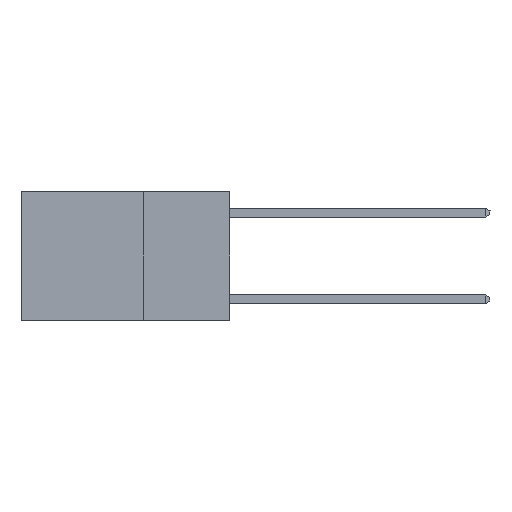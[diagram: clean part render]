
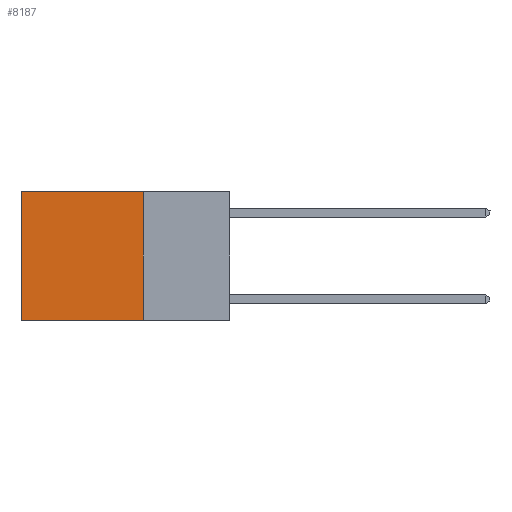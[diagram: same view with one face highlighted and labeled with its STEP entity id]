
A CAD part, left-side view. The second image highlights one B-rep face of the part: STEP entity #8187.
In plain terms, the highlighted planar face has unit normal (-1, 0, 0).
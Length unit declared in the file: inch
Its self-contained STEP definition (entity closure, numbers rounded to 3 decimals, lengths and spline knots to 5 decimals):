
#231 = EDGE_CURVE ( 'NONE', #16517, #11015, #27990, .T. ) ;
#1372 = CARTESIAN_POINT ( 'NONE',  ( 0.2625, 0.6, 0. ) ) ;
#1393 = FACE_OUTER_BOUND ( 'NONE', #3241, .T. ) ;
#1765 = DIRECTION ( 'NONE',  ( 0., 0., -1. ) ) ;
#2202 = CARTESIAN_POINT ( 'NONE',  ( 0.2625, 0.25, 0. ) ) ;
#3241 = EDGE_LOOP ( 'NONE', ( #26690, #14822, #8175, #23675 ) ) ;
#3537 = DIRECTION ( 'NONE',  ( 1., 0., 0. ) ) ;
#3926 = LINE ( 'NONE', #11166, #18707 ) ;
#4234 = DIRECTION ( 'NONE',  ( 0., 1., 0. ) ) ;
#4394 = LINE ( 'NONE', #10884, #12597 ) ;
#5164 = EDGE_CURVE ( 'NONE', #9583, #11015, #3926, .T. ) ;
#5577 = VERTEX_POINT ( 'NONE', #21201 ) ;
#7456 = EDGE_CURVE ( 'NONE', #5577, #16517, #27676, .T. ) ;
#8175 = ORIENTED_EDGE ( 'NONE', *, *, #7456, .F. ) ;
#8187 = ADVANCED_FACE ( 'NONE', ( #1393 ), #22069, .F. ) ;
#9035 = VECTOR ( 'NONE', #11753, 39.37008 ) ;
#9583 = VERTEX_POINT ( 'NONE', #1372 ) ;
#10884 = CARTESIAN_POINT ( 'NONE',  ( 0.2625, 0.25, 0. ) ) ;
#11015 = VERTEX_POINT ( 'NONE', #20175 ) ;
#11166 = CARTESIAN_POINT ( 'NONE',  ( 0.2625, 0.6, 0. ) ) ;
#11753 = DIRECTION ( 'NONE',  ( 0., 0., -1. ) ) ;
#12597 = VECTOR ( 'NONE', #13780, 39.37008 ) ;
#13780 = DIRECTION ( 'NONE',  ( 0., 1., 0. ) ) ;
#14822 = ORIENTED_EDGE ( 'NONE', *, *, #231, .F. ) ;
#15848 = EDGE_CURVE ( 'NONE', #5577, #9583, #4394, .T. ) ;
#16517 = VERTEX_POINT ( 'NONE', #27029 ) ;
#18707 = VECTOR ( 'NONE', #1765, 39.37008 ) ;
#20175 = CARTESIAN_POINT ( 'NONE',  ( 0.2625, 0.6, -0.37 ) ) ;
#20874 = CARTESIAN_POINT ( 'NONE',  ( 0.2625, 0.25, -0.37 ) ) ;
#21201 = CARTESIAN_POINT ( 'NONE',  ( 0.2625, 0.25, 0. ) ) ;
#22069 = PLANE ( 'NONE',  #28748 ) ;
#23675 = ORIENTED_EDGE ( 'NONE', *, *, #15848, .T. ) ;
#24674 = CARTESIAN_POINT ( 'NONE',  ( 0.2625, 0.25, 0. ) ) ;
#25908 = VECTOR ( 'NONE', #4234, 39.37008 ) ;
#26690 = ORIENTED_EDGE ( 'NONE', *, *, #5164, .T. ) ;
#27005 = DIRECTION ( 'NONE',  ( 0., 0., -1. ) ) ;
#27029 = CARTESIAN_POINT ( 'NONE',  ( 0.2625, 0.25, -0.37 ) ) ;
#27676 = LINE ( 'NONE', #2202, #9035 ) ;
#27990 = LINE ( 'NONE', #20874, #25908 ) ;
#28748 = AXIS2_PLACEMENT_3D ( 'NONE', #24674, #3537, #27005 ) ;
